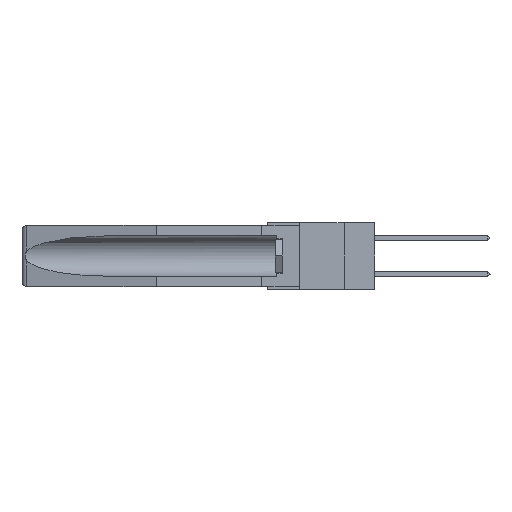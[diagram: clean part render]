
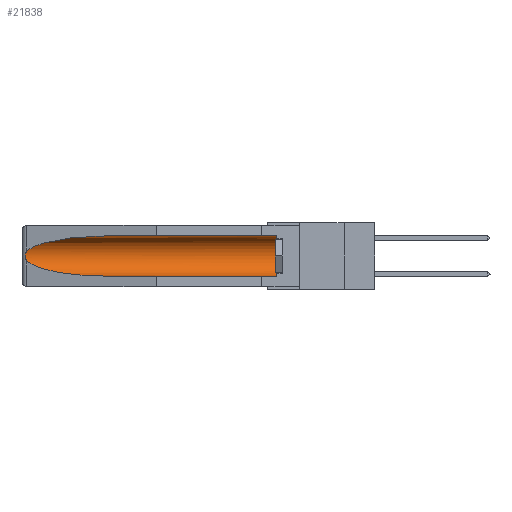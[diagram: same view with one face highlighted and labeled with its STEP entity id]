
A CAD part, left-side view. The second image highlights one B-rep face of the part: STEP entity #21838.
In plain terms, the highlighted cylindrical face has radius 2.857 mm (diameter 5.715 mm), a partial arc.
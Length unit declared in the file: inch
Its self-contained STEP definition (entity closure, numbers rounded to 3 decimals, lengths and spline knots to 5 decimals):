
#36 = CARTESIAN_POINT ( 'NONE',  ( 0.2675, 1.53308, -0.16763 ) ) ;
#71 = CARTESIAN_POINT ( 'NONE',  ( 0.25451, 1.48313, -0.09465 ) ) ;
#585 = CARTESIAN_POINT ( 'NONE',  ( 0.155, -0.30754, -0.059 ) ) ;
#1838 = EDGE_CURVE ( 'NONE', #25481, #29397, #29630, .T. ) ;
#2301 = CARTESIAN_POINT ( 'NONE',  ( 0.155, 1.07973, -0.059 ) ) ;
#2413 = CARTESIAN_POINT ( 'NONE',  ( 0.21114, 1.30732, -0.059 ) ) ;
#2793 = DIRECTION ( 'NONE',  ( 0., 0., 1. ) ) ;
#2838 = EDGE_CURVE ( 'NONE', #7763, #22859, #28684, .T. ) ;
#3047 = CARTESIAN_POINT ( 'NONE',  ( 0.155, 1.07973, -0.059 ) ) ;
#3712 = EDGE_LOOP ( 'NONE', ( #22200, #23204, #14730, #4618, #22771, #28892 ) ) ;
#4462 = VECTOR ( 'NONE', #5525, 39.37008 ) ;
#4472 = CIRCLE ( 'NONE', #15050, 0.1125 ) ;
#4618 = ORIENTED_EDGE ( 'NONE', *, *, #28270, .F. ) ;
#5006 = VERTEX_POINT ( 'NONE', #30554 ) ;
#5525 = DIRECTION ( 'NONE',  ( 0., 1., 0. ) ) ;
#6299 = CARTESIAN_POINT ( 'NONE',  ( 0.155, 0.126, -0.059 ) ) ;
#7002 = CARTESIAN_POINT ( 'NONE',  ( 0.26537, 1.52718, -0.19328 ) ) ;
#7216 = CARTESIAN_POINT ( 'NONE',  ( 0.2673, 1.5327, -0.16383 ) ) ;
#7422 = CARTESIAN_POINT ( 'NONE',  ( 0.2673, 1.53269, -0.17917 ) ) ;
#7763 = VERTEX_POINT ( 'NONE', #18589 ) ;
#8475 = EDGE_CURVE ( 'NONE', #29284, #25481, #10874, .T. ) ;
#9560 = CARTESIAN_POINT ( 'NONE',  ( 0.26654, 1.53092, -0.15636 ) ) ;
#9857 = CARTESIAN_POINT ( 'NONE',  ( 0.26655, 1.53094, -0.18657 ) ) ;
#10874 = LINE ( 'NONE', #585, #4462 ) ;
#11607 = VECTOR ( 'NONE', #24341, 39.37008 ) ;
#11742 = AXIS2_PLACEMENT_3D ( 'NONE', #16611, #14197, #14294 ) ;
#11863 = CARTESIAN_POINT ( 'NONE',  ( 0.155, 1.07973, -0.284 ) ) ;
#12717 = EDGE_CURVE ( 'NONE', #29397, #7763, #21683, .T. ) ;
#14197 = DIRECTION ( 'NONE',  ( 0., 1., 0. ) ) ;
#14294 = DIRECTION ( 'NONE',  ( 0., 0., 1. ) ) ;
#14624 = CYLINDRICAL_SURFACE ( 'NONE', #11742, 0.1125 ) ;
#14730 = ORIENTED_EDGE ( 'NONE', *, *, #2838, .T. ) ;
#15050 = AXIS2_PLACEMENT_3D ( 'NONE', #19608, #19521, #2793 ) ;
#16611 = CARTESIAN_POINT ( 'NONE',  ( 0.155, -0.30754, -0.1715 ) ) ;
#16629 = CARTESIAN_POINT ( 'NONE',  ( 0.26537, 1.52718, -0.14972 ) ) ;
#16842 = CARTESIAN_POINT ( 'NONE',  ( 0.26537, 1.52718, -0.14972 ) ) ;
#17147 = CARTESIAN_POINT ( 'NONE',  ( 0.26537, 1.52718, -0.19328 ) ) ;
#17405 = CARTESIAN_POINT ( 'NONE',  ( 0.155, -0.30754, -0.284 ) ) ;
#17710 = CARTESIAN_POINT ( 'NONE',  ( 0.26537, 1.52718, -0.14972 ) ) ;
#18589 = CARTESIAN_POINT ( 'NONE',  ( 0.26537, 1.52718, -0.19328 ) ) ;
#19288 = CARTESIAN_POINT ( 'NONE',  ( 0.26597, 1.5296, -0.19026 ) ) ;
#19521 = DIRECTION ( 'NONE',  ( 0., -1., 0. ) ) ;
#19608 = CARTESIAN_POINT ( 'NONE',  ( 0.155, 0.126, -0.1715 ) ) ;
#20702 = FACE_OUTER_BOUND ( 'NONE', #3712, .T. ) ;
#21390 = EDGE_CURVE ( 'NONE', #5006, #29284, #4472, .T. ) ;
#21683 = B_SPLINE_CURVE_WITH_KNOTS ( 'NONE', 3,
 ( #16842, #29022, #9560, #7216, #36, #26487, #7422, #9857, #19288, #17147 ),
 .UNSPECIFIED., .F., .F.,
 ( 4, 2, 2, 2, 4 ),
 ( 0., 0.00029, 0.00058, 0.00087, 0.00117 ),
 .UNSPECIFIED. ) ;
#21838 = ADVANCED_FACE ( 'NONE', ( #20702 ), #14624, .F. ) ;
#22200 = ORIENTED_EDGE ( 'NONE', *, *, #1838, .T. ) ;
#22208 = CARTESIAN_POINT ( 'NONE',  ( 0.155, 1.07973, -0.284 ) ) ;
#22771 = ORIENTED_EDGE ( 'NONE', *, *, #21390, .T. ) ;
#22859 = VERTEX_POINT ( 'NONE', #22208 ) ;
#23204 = ORIENTED_EDGE ( 'NONE', *, *, #12717, .T. ) ;
#24341 = DIRECTION ( 'NONE',  ( 0., 1., 0. ) ) ;
#25481 = VERTEX_POINT ( 'NONE', #3047 ) ;
#26374 = CARTESIAN_POINT ( 'NONE',  ( 0.21114, 1.30732, -0.284 ) ) ;
#26487 = CARTESIAN_POINT ( 'NONE',  ( 0.2675, 1.53308, -0.17534 ) ) ;
#28270 = EDGE_CURVE ( 'NONE', #5006, #22859, #29053, .T. ) ;
#28684 =( BOUNDED_CURVE ( )  B_SPLINE_CURVE ( 3, ( #7002, #29008, #26374, #11863 ),
 .UNSPECIFIED., .F., .F. ) 
 B_SPLINE_CURVE_WITH_KNOTS ( ( 4, 4 ),
 ( 0.1948, 1.5708 ),
 .UNSPECIFIED. ) 
 CURVE ( )  GEOMETRIC_REPRESENTATION_ITEM ( )  RATIONAL_B_SPLINE_CURVE ( ( 1., 0.848, 0.848, 1. ) ) 
 REPRESENTATION_ITEM ( '' )  );
#28892 = ORIENTED_EDGE ( 'NONE', *, *, #8475, .T. ) ;
#29008 = CARTESIAN_POINT ( 'NONE',  ( 0.25451, 1.48313, -0.24835 ) ) ;
#29022 = CARTESIAN_POINT ( 'NONE',  ( 0.26597, 1.52961, -0.15275 ) ) ;
#29053 = LINE ( 'NONE', #17405, #11607 ) ;
#29284 = VERTEX_POINT ( 'NONE', #6299 ) ;
#29397 = VERTEX_POINT ( 'NONE', #16629 ) ;
#29630 =( BOUNDED_CURVE ( )  B_SPLINE_CURVE ( 3, ( #2301, #2413, #71, #17710 ),
 .UNSPECIFIED., .F., .F. ) 
 B_SPLINE_CURVE_WITH_KNOTS ( ( 4, 4 ),
 ( 4.71239, 6.08839 ),
 .UNSPECIFIED. ) 
 CURVE ( )  GEOMETRIC_REPRESENTATION_ITEM ( )  RATIONAL_B_SPLINE_CURVE ( ( 1., 0.848, 0.848, 1. ) ) 
 REPRESENTATION_ITEM ( '' )  );
#30554 = CARTESIAN_POINT ( 'NONE',  ( 0.155, 0.126, -0.284 ) ) ;
